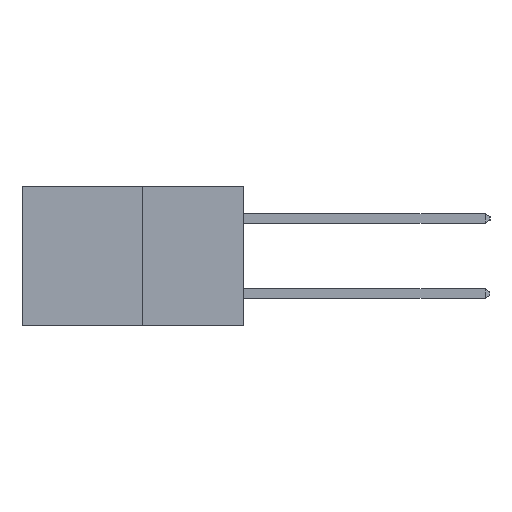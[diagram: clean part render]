
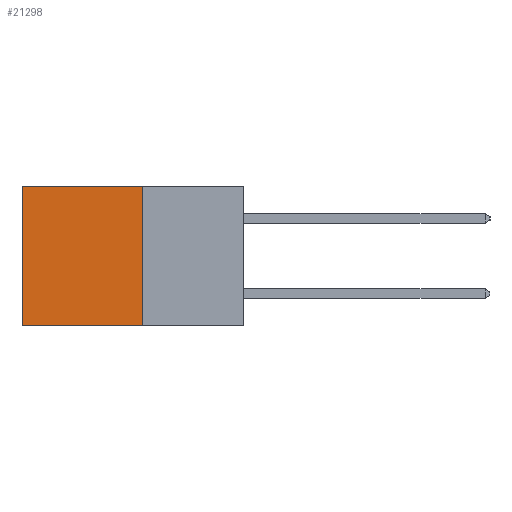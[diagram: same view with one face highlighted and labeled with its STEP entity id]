
A CAD part, left-side view. The second image highlights one B-rep face of the part: STEP entity #21298.
In plain terms, the highlighted planar face has unit normal (-1, 0, 0).
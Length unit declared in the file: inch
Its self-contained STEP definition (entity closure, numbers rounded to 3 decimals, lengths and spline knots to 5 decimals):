
#822 = CARTESIAN_POINT ( 'NONE',  ( 0.277, 0.27, -0.37 ) ) ;
#887 = VECTOR ( 'NONE', #9269, 39.37008 ) ;
#944 = CARTESIAN_POINT ( 'NONE',  ( 0.277, 0.27, -0.37 ) ) ;
#1985 = VERTEX_POINT ( 'NONE', #19529 ) ;
#2865 = EDGE_LOOP ( 'NONE', ( #6902, #7321, #11881, #3223 ) ) ;
#3188 = LINE ( 'NONE', #9686, #3725 ) ;
#3223 = ORIENTED_EDGE ( 'NONE', *, *, #14280, .T. ) ;
#3725 = VECTOR ( 'NONE', #11372, 39.37008 ) ;
#4315 = CARTESIAN_POINT ( 'NONE',  ( 0.277, 0.59, -0.37 ) ) ;
#4899 = LINE ( 'NONE', #10617, #9104 ) ;
#5178 = VECTOR ( 'NONE', #6090, 39.37008 ) ;
#5238 = FACE_OUTER_BOUND ( 'NONE', #2865, .T. ) ;
#5594 = EDGE_CURVE ( 'NONE', #19734, #8800, #4899, .T. ) ;
#6090 = DIRECTION ( 'NONE',  ( 0., 1., 0. ) ) ;
#6902 = ORIENTED_EDGE ( 'NONE', *, *, #5594, .T. ) ;
#7254 = DIRECTION ( 'NONE',  ( 0., 0., -1. ) ) ;
#7321 = ORIENTED_EDGE ( 'NONE', *, *, #11018, .F. ) ;
#8800 = VERTEX_POINT ( 'NONE', #4315 ) ;
#9104 = VECTOR ( 'NONE', #7254, 39.37008 ) ;
#9269 = DIRECTION ( 'NONE',  ( 0., 0., -1. ) ) ;
#9644 = LINE ( 'NONE', #944, #5178 ) ;
#9654 = DIRECTION ( 'NONE',  ( 1., 0., 0. ) ) ;
#9686 = CARTESIAN_POINT ( 'NONE',  ( 0.277, 0.27, 0. ) ) ;
#10617 = CARTESIAN_POINT ( 'NONE',  ( 0.277, 0.59, -0.37 ) ) ;
#11018 = EDGE_CURVE ( 'NONE', #11223, #8800, #9644, .T. ) ;
#11223 = VERTEX_POINT ( 'NONE', #16393 ) ;
#11372 = DIRECTION ( 'NONE',  ( 0., 1., 0. ) ) ;
#11881 = ORIENTED_EDGE ( 'NONE', *, *, #12359, .F. ) ;
#12359 = EDGE_CURVE ( 'NONE', #1985, #11223, #18591, .T. ) ;
#13678 = CARTESIAN_POINT ( 'NONE',  ( 0.277, 0.59, 0. ) ) ;
#14280 = EDGE_CURVE ( 'NONE', #1985, #19734, #3188, .T. ) ;
#16393 = CARTESIAN_POINT ( 'NONE',  ( 0.277, 0.27, -0.37 ) ) ;
#18591 = LINE ( 'NONE', #822, #887 ) ;
#19346 = AXIS2_PLACEMENT_3D ( 'NONE', #19469, #9654, #21050 ) ;
#19404 = PLANE ( 'NONE',  #19346 ) ;
#19469 = CARTESIAN_POINT ( 'NONE',  ( 0.277, 0.27, -0.37 ) ) ;
#19529 = CARTESIAN_POINT ( 'NONE',  ( 0.277, 0.27, 0. ) ) ;
#19734 = VERTEX_POINT ( 'NONE', #13678 ) ;
#21050 = DIRECTION ( 'NONE',  ( 0., 0., -1. ) ) ;
#21298 = ADVANCED_FACE ( 'NONE', ( #5238 ), #19404, .F. ) ;
